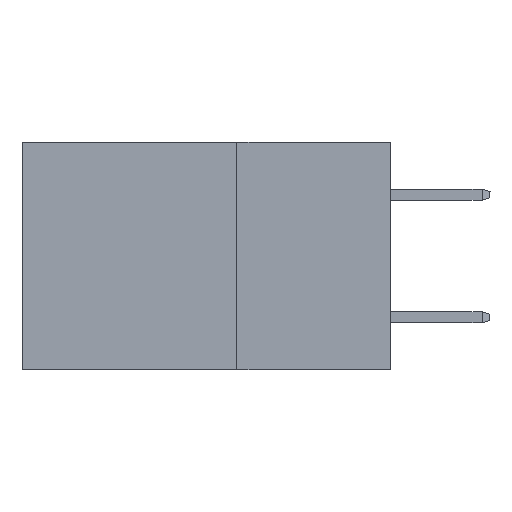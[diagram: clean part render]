
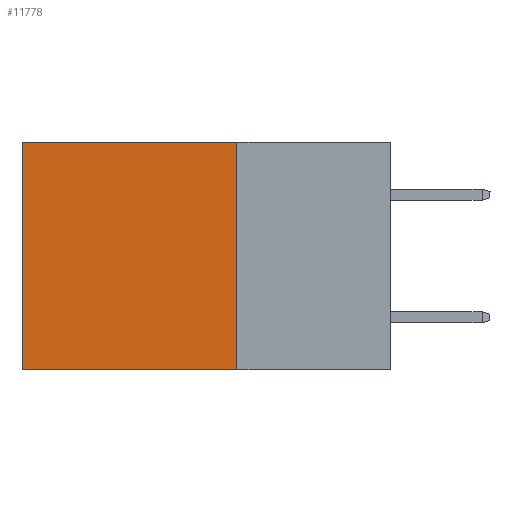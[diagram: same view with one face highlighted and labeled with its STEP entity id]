
A CAD part, left-side view. The second image highlights one B-rep face of the part: STEP entity #11778.
In plain terms, the highlighted planar face has unit normal (-1, 0, 0).
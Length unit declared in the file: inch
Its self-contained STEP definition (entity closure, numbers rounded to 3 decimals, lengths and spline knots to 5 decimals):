
#442 = DIRECTION ( 'NONE',  ( 0., 0., -1. ) ) ;
#585 = CARTESIAN_POINT ( 'NONE',  ( 0.2875, 0.25, 0. ) ) ;
#1110 = EDGE_CURVE ( 'NONE', #27753, #11870, #16430, .T. ) ;
#2324 = FACE_OUTER_BOUND ( 'NONE', #17253, .T. ) ;
#4510 = DIRECTION ( 'NONE',  ( 0., 0., -1. ) ) ;
#5574 = CARTESIAN_POINT ( 'NONE',  ( 0.2875, 0.25, 0. ) ) ;
#6161 = ORIENTED_EDGE ( 'NONE', *, *, #1110, .F. ) ;
#6259 = AXIS2_PLACEMENT_3D ( 'NONE', #5574, #29866, #13706 ) ;
#9036 = ORIENTED_EDGE ( 'NONE', *, *, #27094, .T. ) ;
#11102 = ORIENTED_EDGE ( 'NONE', *, *, #15307, .T. ) ;
#11193 = CARTESIAN_POINT ( 'NONE',  ( 0.2875, 0.25, 0. ) ) ;
#11426 = VECTOR ( 'NONE', #32845, 39.37008 ) ;
#11778 = ADVANCED_FACE ( 'NONE', ( #2324 ), #29740, .F. ) ;
#11870 = VERTEX_POINT ( 'NONE', #22328 ) ;
#12588 = CARTESIAN_POINT ( 'NONE',  ( 0.2875, 0.25, -0.37 ) ) ;
#13706 = DIRECTION ( 'NONE',  ( 0., 0., -1. ) ) ;
#14940 = VECTOR ( 'NONE', #4510, 39.37008 ) ;
#15307 = EDGE_CURVE ( 'NONE', #26751, #26458, #22132, .T. ) ;
#15579 = VECTOR ( 'NONE', #442, 39.37008 ) ;
#16178 = ORIENTED_EDGE ( 'NONE', *, *, #28887, .F. ) ;
#16430 = LINE ( 'NONE', #11193, #15579 ) ;
#17253 = EDGE_LOOP ( 'NONE', ( #11102, #16178, #6161, #9036 ) ) ;
#18459 = VECTOR ( 'NONE', #34106, 39.37008 ) ;
#18591 = LINE ( 'NONE', #585, #11426 ) ;
#22132 = LINE ( 'NONE', #26099, #14940 ) ;
#22328 = CARTESIAN_POINT ( 'NONE',  ( 0.2875, 0.25, -0.37 ) ) ;
#26099 = CARTESIAN_POINT ( 'NONE',  ( 0.2875, 0.6, 0. ) ) ;
#26326 = CARTESIAN_POINT ( 'NONE',  ( 0.2875, 0.6, 0. ) ) ;
#26458 = VERTEX_POINT ( 'NONE', #27756 ) ;
#26751 = VERTEX_POINT ( 'NONE', #26326 ) ;
#27094 = EDGE_CURVE ( 'NONE', #27753, #26751, #18591, .T. ) ;
#27753 = VERTEX_POINT ( 'NONE', #32798 ) ;
#27756 = CARTESIAN_POINT ( 'NONE',  ( 0.2875, 0.6, -0.37 ) ) ;
#28887 = EDGE_CURVE ( 'NONE', #11870, #26458, #32744, .T. ) ;
#29740 = PLANE ( 'NONE',  #6259 ) ;
#29866 = DIRECTION ( 'NONE',  ( 1., 0., 0. ) ) ;
#32744 = LINE ( 'NONE', #12588, #18459 ) ;
#32798 = CARTESIAN_POINT ( 'NONE',  ( 0.2875, 0.25, 0. ) ) ;
#32845 = DIRECTION ( 'NONE',  ( 0., 1., 0. ) ) ;
#34106 = DIRECTION ( 'NONE',  ( 0., 1., 0. ) ) ;
